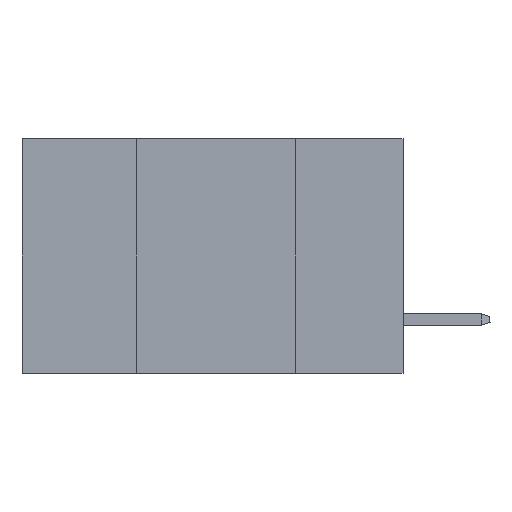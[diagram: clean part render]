
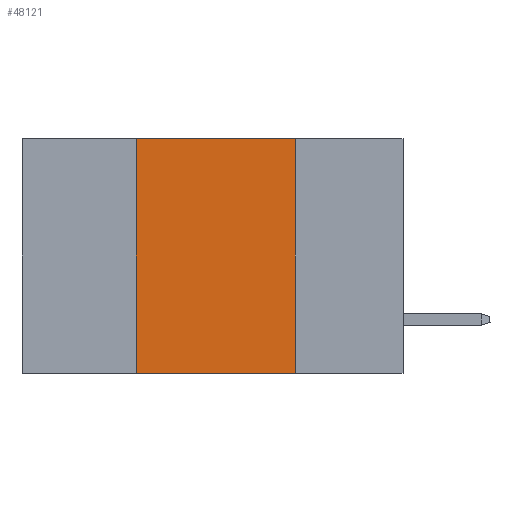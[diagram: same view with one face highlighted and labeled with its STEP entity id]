
A CAD part, left-side view. The second image highlights one B-rep face of the part: STEP entity #48121.
In plain terms, the highlighted planar face has unit normal (-1, 0, 0).
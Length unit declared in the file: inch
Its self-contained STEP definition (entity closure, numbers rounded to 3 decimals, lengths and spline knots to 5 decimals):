
#312 = DIRECTION ( 'NONE',  ( 0., 0., 1. ) ) ;
#1524 = LINE ( 'NONE', #13082, #9239 ) ;
#1828 = DIRECTION ( 'NONE',  ( 0., -1., 0. ) ) ;
#3282 = VERTEX_POINT ( 'NONE', #32278 ) ;
#9239 = VECTOR ( 'NONE', #24138, 39.37008 ) ;
#10261 = CARTESIAN_POINT ( 'NONE',  ( 0., 0.17, 0. ) ) ;
#11106 = VECTOR ( 'NONE', #1828, 39.37008 ) ;
#13082 = CARTESIAN_POINT ( 'NONE',  ( 0., 0.6, -0.37 ) ) ;
#14486 = ORIENTED_EDGE ( 'NONE', *, *, #20205, .F. ) ;
#14655 = CARTESIAN_POINT ( 'NONE',  ( 0., 0.42, 0. ) ) ;
#17810 = DIRECTION ( 'NONE',  ( 0., 0., -1. ) ) ;
#18567 = LINE ( 'NONE', #10261, #26512 ) ;
#19186 = ORIENTED_EDGE ( 'NONE', *, *, #22761, .T. ) ;
#19823 = ORIENTED_EDGE ( 'NONE', *, *, #20567, .F. ) ;
#20205 = EDGE_CURVE ( 'NONE', #46812, #27392, #18567, .T. ) ;
#20567 = EDGE_CURVE ( 'NONE', #26365, #3282, #41283, .T. ) ;
#20939 = LINE ( 'NONE', #40271, #11106 ) ;
#22761 = EDGE_CURVE ( 'NONE', #26365, #27392, #1524, .T. ) ;
#24138 = DIRECTION ( 'NONE',  ( 0., -1., 0. ) ) ;
#24650 = ORIENTED_EDGE ( 'NONE', *, *, #39891, .F. ) ;
#26365 = VERTEX_POINT ( 'NONE', #29510 ) ;
#26512 = VECTOR ( 'NONE', #17810, 39.37008 ) ;
#27379 = VECTOR ( 'NONE', #312, 39.37008 ) ;
#27392 = VERTEX_POINT ( 'NONE', #40088 ) ;
#29290 = CARTESIAN_POINT ( 'NONE',  ( 0., 0.6, 0. ) ) ;
#29510 = CARTESIAN_POINT ( 'NONE',  ( 0., 0.42, -0.37 ) ) ;
#32278 = CARTESIAN_POINT ( 'NONE',  ( 0., 0.42, 0. ) ) ;
#32549 = EDGE_LOOP ( 'NONE', ( #14486, #24650, #19823, #19186 ) ) ;
#36349 = DIRECTION ( 'NONE',  ( 1., 0., 0. ) ) ;
#39891 = EDGE_CURVE ( 'NONE', #3282, #46812, #20939, .T. ) ;
#40088 = CARTESIAN_POINT ( 'NONE',  ( 0., 0.17, -0.37 ) ) ;
#40271 = CARTESIAN_POINT ( 'NONE',  ( 0., 0.6, 0. ) ) ;
#41283 = LINE ( 'NONE', #14655, #27379 ) ;
#44124 = DIRECTION ( 'NONE',  ( 0., 0., -1. ) ) ;
#44620 = PLANE ( 'NONE',  #46384 ) ;
#46384 = AXIS2_PLACEMENT_3D ( 'NONE', #29290, #36349, #44124 ) ;
#46812 = VERTEX_POINT ( 'NONE', #47350 ) ;
#47350 = CARTESIAN_POINT ( 'NONE',  ( 0., 0.17, 0. ) ) ;
#47920 = FACE_OUTER_BOUND ( 'NONE', #32549, .T. ) ;
#48121 = ADVANCED_FACE ( 'NONE', ( #47920 ), #44620, .F. ) ;
